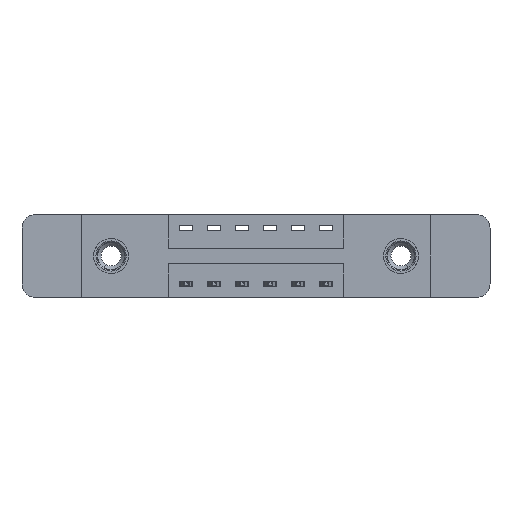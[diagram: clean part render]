
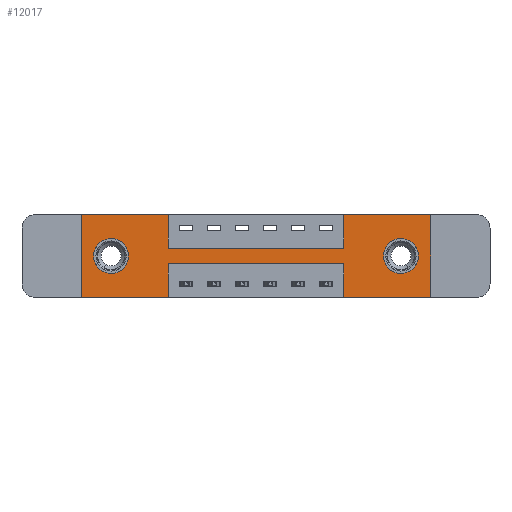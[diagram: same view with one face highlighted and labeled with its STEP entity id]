
A CAD part, front view. The second image highlights one B-rep face of the part: STEP entity #12017.
In plain terms, the highlighted planar face has unit normal (0, -1, 0).
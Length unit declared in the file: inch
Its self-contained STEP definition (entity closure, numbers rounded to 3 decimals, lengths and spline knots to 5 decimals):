
#14 = ORIENTED_EDGE ( 'NONE', *, *, #6721, .F. ) ;
#34 = ORIENTED_EDGE ( 'NONE', *, *, #2247, .T. ) ;
#259 = CARTESIAN_POINT ( 'NONE',  ( 0.3875, 0., -0.22 ) ) ;
#317 = CARTESIAN_POINT ( 'NONE',  ( 1.1725, 0., -0.37 ) ) ;
#361 = VECTOR ( 'NONE', #1785, 39.37008 ) ;
#550 = CARTESIAN_POINT ( 'NONE',  ( 1.4275, 0., -0.185 ) ) ;
#566 = VERTEX_POINT ( 'NONE', #5964 ) ;
#578 = EDGE_CURVE ( 'NONE', #9493, #10327, #4666, .T. ) ;
#612 = CIRCLE ( 'NONE', #4932, 0.078 ) ;
#656 = EDGE_CURVE ( 'NONE', #12654, #7962, #810, .T. ) ;
#665 = CARTESIAN_POINT ( 'NONE',  ( 0., 0., -0.37 ) ) ;
#697 = ORIENTED_EDGE ( 'NONE', *, *, #3306, .F. ) ;
#716 = EDGE_CURVE ( 'NONE', #566, #11041, #12970, .T. ) ;
#810 = LINE ( 'NONE', #2890, #3967 ) ;
#937 = CARTESIAN_POINT ( 'NONE',  ( 0.3875, 0., 0. ) ) ;
#979 = LINE ( 'NONE', #9876, #8902 ) ;
#1062 = VERTEX_POINT ( 'NONE', #12745 ) ;
#1125 = EDGE_CURVE ( 'NONE', #12758, #566, #13957, .T. ) ;
#1175 = ORIENTED_EDGE ( 'NONE', *, *, #578, .F. ) ;
#1476 = DIRECTION ( 'NONE',  ( 0., 0., -1. ) ) ;
#1559 = DIRECTION ( 'NONE',  ( 0., 0., 1. ) ) ;
#1580 = LINE ( 'NONE', #5928, #12525 ) ;
#1730 = CARTESIAN_POINT ( 'NONE',  ( 1.56, 0., -0.37 ) ) ;
#1758 = CARTESIAN_POINT ( 'NONE',  ( 0., 0., 0. ) ) ;
#1785 = DIRECTION ( 'NONE',  ( 0., 0., -1. ) ) ;
#1817 = CARTESIAN_POINT ( 'NONE',  ( 0.3875, 0., -0.15 ) ) ;
#2005 = CARTESIAN_POINT ( 'NONE',  ( 0., 0., -0.37 ) ) ;
#2247 = EDGE_CURVE ( 'NONE', #12660, #2989, #612, .T. ) ;
#2298 = ORIENTED_EDGE ( 'NONE', *, *, #12638, .F. ) ;
#2335 = EDGE_CURVE ( 'NONE', #2972, #6003, #6537, .T. ) ;
#2427 = CARTESIAN_POINT ( 'NONE',  ( 1.4275, 0., -0.107 ) ) ;
#2616 = AXIS2_PLACEMENT_3D ( 'NONE', #665, #3868, #11457 ) ;
#2736 = FACE_BOUND ( 'NONE', #11551, .T. ) ;
#2769 = EDGE_CURVE ( 'NONE', #6512, #12758, #5814, .T. ) ;
#2817 = CARTESIAN_POINT ( 'NONE',  ( 0., 0., 0. ) ) ;
#2828 = ORIENTED_EDGE ( 'NONE', *, *, #6939, .F. ) ;
#2889 = VERTEX_POINT ( 'NONE', #6375 ) ;
#2890 = CARTESIAN_POINT ( 'NONE',  ( 0., 0., 0. ) ) ;
#2972 = VERTEX_POINT ( 'NONE', #6800 ) ;
#2989 = VERTEX_POINT ( 'NONE', #3312 ) ;
#3001 = LINE ( 'NONE', #937, #361 ) ;
#3054 = CARTESIAN_POINT ( 'NONE',  ( 0.1325, 0., -0.185 ) ) ;
#3306 = EDGE_CURVE ( 'NONE', #7962, #2889, #3001, .T. ) ;
#3312 = CARTESIAN_POINT ( 'NONE',  ( 0.1325, 0., -0.263 ) ) ;
#3440 = EDGE_LOOP ( 'NONE', ( #34, #6169 ) ) ;
#3703 = EDGE_CURVE ( 'NONE', #2989, #12660, #8369, .T. ) ;
#3868 = DIRECTION ( 'NONE',  ( 0., -1., 0. ) ) ;
#3895 = DIRECTION ( 'NONE',  ( 0., 0., -1. ) ) ;
#3945 = DIRECTION ( 'NONE',  ( 1., 0., 0. ) ) ;
#3955 = CARTESIAN_POINT ( 'NONE',  ( 0.3875, 0., -0.37 ) ) ;
#3967 = VECTOR ( 'NONE', #13826, 39.37008 ) ;
#4196 = ORIENTED_EDGE ( 'NONE', *, *, #1125, .F. ) ;
#4284 = DIRECTION ( 'NONE',  ( -1., 0., 0. ) ) ;
#4501 = EDGE_CURVE ( 'NONE', #11041, #8303, #11871, .T. ) ;
#4666 = LINE ( 'NONE', #11257, #8339 ) ;
#4868 = FACE_OUTER_BOUND ( 'NONE', #5307, .T. ) ;
#4932 = AXIS2_PLACEMENT_3D ( 'NONE', #7129, #8342, #11548 ) ;
#5307 = EDGE_LOOP ( 'NONE', ( #1175, #11538, #2298, #9460, #9870, #4196, #9729, #2828, #697, #10733, #13537, #14 ) ) ;
#5317 = DIRECTION ( 'NONE',  ( -1., 0., 0. ) ) ;
#5350 = VECTOR ( 'NONE', #11895, 39.37008 ) ;
#5627 = VECTOR ( 'NONE', #4284, 39.37008 ) ;
#5700 = EDGE_CURVE ( 'NONE', #1062, #12654, #13627, .T. ) ;
#5814 = LINE ( 'NONE', #9264, #9311 ) ;
#5928 = CARTESIAN_POINT ( 'NONE',  ( 0.3875, 0., -0.22 ) ) ;
#5964 = CARTESIAN_POINT ( 'NONE',  ( 1.56, 0., 0. ) ) ;
#6003 = VERTEX_POINT ( 'NONE', #2427 ) ;
#6060 = VECTOR ( 'NONE', #9401, 39.37008 ) ;
#6119 = VECTOR ( 'NONE', #13708, 39.37008 ) ;
#6169 = ORIENTED_EDGE ( 'NONE', *, *, #3703, .T. ) ;
#6245 = VECTOR ( 'NONE', #1559, 39.37008 ) ;
#6375 = CARTESIAN_POINT ( 'NONE',  ( 0.3875, 0., -0.15 ) ) ;
#6453 = CARTESIAN_POINT ( 'NONE',  ( 1.4275, 0., -0.185 ) ) ;
#6512 = VERTEX_POINT ( 'NONE', #12505 ) ;
#6537 = CIRCLE ( 'NONE', #13466, 0.078 ) ;
#6721 = EDGE_CURVE ( 'NONE', #10327, #1062, #979, .T. ) ;
#6800 = CARTESIAN_POINT ( 'NONE',  ( 1.4275, 0., -0.263 ) ) ;
#6939 = EDGE_CURVE ( 'NONE', #2889, #6512, #11688, .T. ) ;
#7129 = CARTESIAN_POINT ( 'NONE',  ( 0.1325, 0., -0.185 ) ) ;
#7241 = PLANE ( 'NONE',  #2616 ) ;
#7269 = LINE ( 'NONE', #8137, #6245 ) ;
#7420 = DIRECTION ( 'NONE',  ( 0., 1., 0. ) ) ;
#7445 = CARTESIAN_POINT ( 'NONE',  ( 0., 0., 0. ) ) ;
#7461 = CARTESIAN_POINT ( 'NONE',  ( 1.56, 0., 0. ) ) ;
#7813 = CARTESIAN_POINT ( 'NONE',  ( 1.1725, 0., -0.22 ) ) ;
#7962 = VERTEX_POINT ( 'NONE', #11414 ) ;
#7981 = ORIENTED_EDGE ( 'NONE', *, *, #8203, .T. ) ;
#8137 = CARTESIAN_POINT ( 'NONE',  ( 1.1725, 0., -0.37 ) ) ;
#8185 = DIRECTION ( 'NONE',  ( 0., 0., 1. ) ) ;
#8203 = EDGE_CURVE ( 'NONE', #6003, #2972, #13342, .T. ) ;
#8303 = VERTEX_POINT ( 'NONE', #317 ) ;
#8339 = VECTOR ( 'NONE', #1476, 39.37008 ) ;
#8342 = DIRECTION ( 'NONE',  ( 0., 1., 0. ) ) ;
#8369 = CIRCLE ( 'NONE', #9300, 0.078 ) ;
#8627 = DIRECTION ( 'NONE',  ( 0., 1., 0. ) ) ;
#8846 = DIRECTION ( 'NONE',  ( 0., 0., -1. ) ) ;
#8902 = VECTOR ( 'NONE', #5317, 39.37008 ) ;
#9264 = CARTESIAN_POINT ( 'NONE',  ( 1.1725, 0., 0. ) ) ;
#9300 = AXIS2_PLACEMENT_3D ( 'NONE', #3054, #7420, #11849 ) ;
#9311 = VECTOR ( 'NONE', #8185, 39.37008 ) ;
#9401 = DIRECTION ( 'NONE',  ( 1., 0., 0. ) ) ;
#9460 = ORIENTED_EDGE ( 'NONE', *, *, #4501, .F. ) ;
#9493 = VERTEX_POINT ( 'NONE', #259 ) ;
#9729 = ORIENTED_EDGE ( 'NONE', *, *, #2769, .F. ) ;
#9870 = ORIENTED_EDGE ( 'NONE', *, *, #716, .F. ) ;
#9876 = CARTESIAN_POINT ( 'NONE',  ( 0., 0., -0.37 ) ) ;
#10098 = CARTESIAN_POINT ( 'NONE',  ( 1.1725, 0., 0. ) ) ;
#10112 = AXIS2_PLACEMENT_3D ( 'NONE', #6453, #8627, #8846 ) ;
#10194 = DIRECTION ( 'NONE',  ( -1., 0., 0. ) ) ;
#10327 = VERTEX_POINT ( 'NONE', #3955 ) ;
#10571 = FACE_BOUND ( 'NONE', #3440, .T. ) ;
#10733 = ORIENTED_EDGE ( 'NONE', *, *, #656, .F. ) ;
#11041 = VERTEX_POINT ( 'NONE', #1730 ) ;
#11257 = CARTESIAN_POINT ( 'NONE',  ( 0.3875, 0., -0.37 ) ) ;
#11414 = CARTESIAN_POINT ( 'NONE',  ( 0.3875, 0., 0. ) ) ;
#11457 = DIRECTION ( 'NONE',  ( 0., 0., -1. ) ) ;
#11538 = ORIENTED_EDGE ( 'NONE', *, *, #12533, .F. ) ;
#11548 = DIRECTION ( 'NONE',  ( 0., 0., 1. ) ) ;
#11551 = EDGE_LOOP ( 'NONE', ( #7981, #12074 ) ) ;
#11688 = LINE ( 'NONE', #1817, #12859 ) ;
#11695 = CARTESIAN_POINT ( 'NONE',  ( 0.1325, 0., -0.107 ) ) ;
#11849 = DIRECTION ( 'NONE',  ( 0., 0., 1. ) ) ;
#11871 = LINE ( 'NONE', #2005, #5627 ) ;
#11895 = DIRECTION ( 'NONE',  ( 0., 0., -1. ) ) ;
#11965 = VERTEX_POINT ( 'NONE', #7813 ) ;
#12017 = ADVANCED_FACE ( 'NONE', ( #2736, #10571, #4868 ), #7241, .T. ) ;
#12074 = ORIENTED_EDGE ( 'NONE', *, *, #2335, .T. ) ;
#12489 = DIRECTION ( 'NONE',  ( 0., 1., 0. ) ) ;
#12505 = CARTESIAN_POINT ( 'NONE',  ( 1.1725, 0., -0.15 ) ) ;
#12525 = VECTOR ( 'NONE', #10194, 39.37008 ) ;
#12533 = EDGE_CURVE ( 'NONE', #11965, #9493, #1580, .T. ) ;
#12638 = EDGE_CURVE ( 'NONE', #8303, #11965, #7269, .T. ) ;
#12654 = VERTEX_POINT ( 'NONE', #1758 ) ;
#12660 = VERTEX_POINT ( 'NONE', #11695 ) ;
#12745 = CARTESIAN_POINT ( 'NONE',  ( 0., 0., -0.37 ) ) ;
#12758 = VERTEX_POINT ( 'NONE', #10098 ) ;
#12859 = VECTOR ( 'NONE', #3945, 39.37008 ) ;
#12970 = LINE ( 'NONE', #7461, #5350 ) ;
#13342 = CIRCLE ( 'NONE', #10112, 0.078 ) ;
#13466 = AXIS2_PLACEMENT_3D ( 'NONE', #550, #12489, #3895 ) ;
#13537 = ORIENTED_EDGE ( 'NONE', *, *, #5700, .F. ) ;
#13627 = LINE ( 'NONE', #2817, #6119 ) ;
#13708 = DIRECTION ( 'NONE',  ( 0., 0., 1. ) ) ;
#13826 = DIRECTION ( 'NONE',  ( 1., 0., 0. ) ) ;
#13957 = LINE ( 'NONE', #7445, #6060 ) ;
